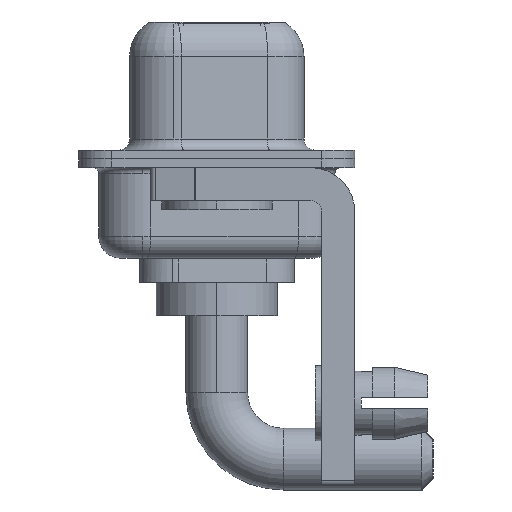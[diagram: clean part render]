
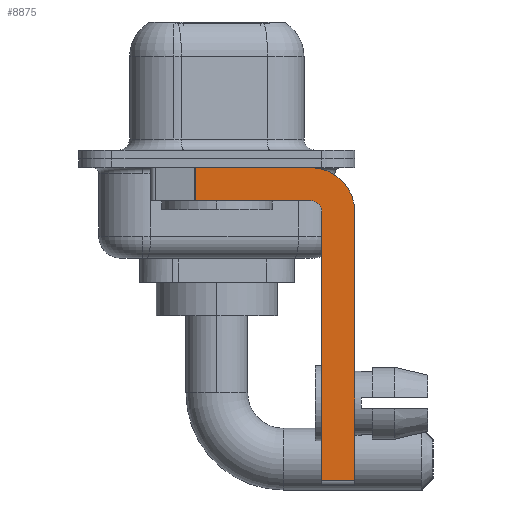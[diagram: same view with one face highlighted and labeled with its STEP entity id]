
A CAD part, left-side view. The second image highlights one B-rep face of the part: STEP entity #8875.
In plain terms, the highlighted planar face has unit normal (-1, 0, 0).
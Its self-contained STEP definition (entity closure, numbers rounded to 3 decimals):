
#11 = VECTOR ( 'NONE', #15070, 1000. ) ;
#226 = CARTESIAN_POINT ( 'NONE',  ( -2.9, -4.25, -2.4 ) ) ;
#414 = LINE ( 'NONE', #12399, #6335 ) ;
#458 = EDGE_CURVE ( 'NONE', #7240, #4676, #15631, .T. ) ;
#977 = EDGE_CURVE ( 'NONE', #4676, #10239, #12393, .T. ) ;
#1040 = DIRECTION ( 'NONE',  ( 0., 0., -1. ) ) ;
#1063 = EDGE_CURVE ( 'NONE', #7240, #3313, #414, .T. ) ;
#1226 = LINE ( 'NONE', #1298, #6947 ) ;
#1298 = CARTESIAN_POINT ( 'NONE',  ( -2.9, -4.25, -1.9 ) ) ;
#1462 = DIRECTION ( 'NONE',  ( 0., 1., 0. ) ) ;
#1628 = EDGE_CURVE ( 'NONE', #7378, #12420, #5485, .T. ) ;
#1643 = EDGE_CURVE ( 'NONE', #10239, #13677, #7795, .T. ) ;
#2261 = DIRECTION ( 'NONE',  ( 0., 0., -1. ) ) ;
#2277 = ORIENTED_EDGE ( 'NONE', *, *, #5719, .F. ) ;
#2289 = CARTESIAN_POINT ( 'NONE',  ( -2.9, 3., -0.4 ) ) ;
#2551 = CARTESIAN_POINT ( 'NONE',  ( -2.9, -4.25, -1.9 ) ) ;
#3209 = LINE ( 'NONE', #13131, #12518 ) ;
#3247 = DIRECTION ( 'NONE',  ( 0., 0., -1. ) ) ;
#3286 = DIRECTION ( 'NONE',  ( 0., -1., 0. ) ) ;
#3313 = VERTEX_POINT ( 'NONE', #6469 ) ;
#3977 = CARTESIAN_POINT ( 'NONE',  ( -2.9, -6.25, -14.55 ) ) ;
#4252 = ORIENTED_EDGE ( 'NONE', *, *, #1628, .F. ) ;
#4577 = ORIENTED_EDGE ( 'NONE', *, *, #7951, .T. ) ;
#4676 = VERTEX_POINT ( 'NONE', #7534 ) ;
#4721 = CARTESIAN_POINT ( 'NONE',  ( -2.9, -4.25, -2.4 ) ) ;
#4760 = DIRECTION ( 'NONE',  ( 0., -1., 0. ) ) ;
#4890 = EDGE_LOOP ( 'NONE', ( #10134, #7682, #13260, #2277, #4252, #4577, #13034, #7913 ) ) ;
#5205 = AXIS2_PLACEMENT_3D ( 'NONE', #226, #7397, #9913 ) ;
#5477 = AXIS2_PLACEMENT_3D ( 'NONE', #12708, #11925, #1040 ) ;
#5485 = LINE ( 'NONE', #14129, #11 ) ;
#5719 = EDGE_CURVE ( 'NONE', #12420, #11117, #12049, .T. ) ;
#6335 = VECTOR ( 'NONE', #7727, 1000. ) ;
#6342 = VECTOR ( 'NONE', #3247, 1000. ) ;
#6469 = CARTESIAN_POINT ( 'NONE',  ( -2.9, 0.978, -1.9 ) ) ;
#6947 = VECTOR ( 'NONE', #1462, 1000. ) ;
#7240 = VERTEX_POINT ( 'NONE', #11110 ) ;
#7378 = VERTEX_POINT ( 'NONE', #7619 ) ;
#7397 = DIRECTION ( 'NONE',  ( -1., 0., 0. ) ) ;
#7534 = CARTESIAN_POINT ( 'NONE',  ( -2.9, -4.25, -0.4 ) ) ;
#7619 = CARTESIAN_POINT ( 'NONE',  ( -2.9, -4.75, -14.55 ) ) ;
#7682 = ORIENTED_EDGE ( 'NONE', *, *, #1063, .T. ) ;
#7727 = DIRECTION ( 'NONE',  ( 0., 0., -1. ) ) ;
#7795 = LINE ( 'NONE', #7866, #6342 ) ;
#7866 = CARTESIAN_POINT ( 'NONE',  ( -2.9, -6.25, -2.4 ) ) ;
#7885 = PLANE ( 'NONE',  #5477 ) ;
#7913 = ORIENTED_EDGE ( 'NONE', *, *, #977, .F. ) ;
#7951 = EDGE_CURVE ( 'NONE', #7378, #13677, #3209, .T. ) ;
#8875 = ADVANCED_FACE ( 'NONE', ( #15093 ), #7885, .F. ) ;
#9913 = DIRECTION ( 'NONE',  ( 0., 0., 1. ) ) ;
#10134 = ORIENTED_EDGE ( 'NONE', *, *, #458, .F. ) ;
#10239 = VERTEX_POINT ( 'NONE', #11385 ) ;
#11110 = CARTESIAN_POINT ( 'NONE',  ( -2.9, 0.978, -0.4 ) ) ;
#11117 = VERTEX_POINT ( 'NONE', #2551 ) ;
#11385 = CARTESIAN_POINT ( 'NONE',  ( -2.9, -6.25, -2.4 ) ) ;
#11725 = CARTESIAN_POINT ( 'NONE',  ( -2.9, -4.75, -2.4 ) ) ;
#11872 = DIRECTION ( 'NONE',  ( 1., 0., 0. ) ) ;
#11925 = DIRECTION ( 'NONE',  ( 1., 0., 0. ) ) ;
#11979 = VECTOR ( 'NONE', #4760, 1000. ) ;
#12049 = CIRCLE ( 'NONE', #5205, 0.5 ) ;
#12393 = CIRCLE ( 'NONE', #15185, 2. ) ;
#12399 = CARTESIAN_POINT ( 'NONE',  ( -2.9, 0.978, -1.9 ) ) ;
#12420 = VERTEX_POINT ( 'NONE', #11725 ) ;
#12518 = VECTOR ( 'NONE', #3286, 1000. ) ;
#12708 = CARTESIAN_POINT ( 'NONE',  ( -2.9, -4.25, -2.4 ) ) ;
#13034 = ORIENTED_EDGE ( 'NONE', *, *, #1643, .F. ) ;
#13095 = EDGE_CURVE ( 'NONE', #11117, #3313, #1226, .T. ) ;
#13131 = CARTESIAN_POINT ( 'NONE',  ( -2.9, -4.25, -14.55 ) ) ;
#13260 = ORIENTED_EDGE ( 'NONE', *, *, #13095, .F. ) ;
#13677 = VERTEX_POINT ( 'NONE', #3977 ) ;
#14129 = CARTESIAN_POINT ( 'NONE',  ( -2.9, -4.75, -14.8 ) ) ;
#15070 = DIRECTION ( 'NONE',  ( 0., 0., 1. ) ) ;
#15093 = FACE_OUTER_BOUND ( 'NONE', #4890, .T. ) ;
#15185 = AXIS2_PLACEMENT_3D ( 'NONE', #4721, #11872, #2261 ) ;
#15631 = LINE ( 'NONE', #2289, #11979 ) ;
